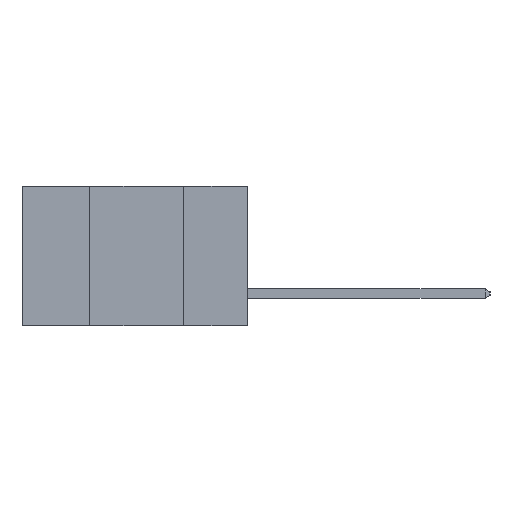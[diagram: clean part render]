
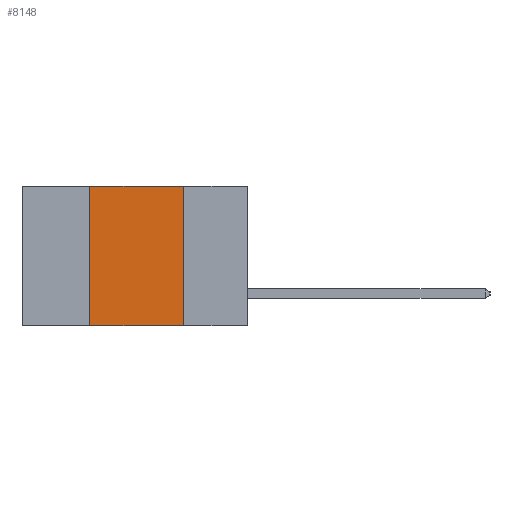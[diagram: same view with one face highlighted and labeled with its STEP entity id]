
A CAD part, left-side view. The second image highlights one B-rep face of the part: STEP entity #8148.
In plain terms, the highlighted planar face has unit normal (-1, 0, 0).
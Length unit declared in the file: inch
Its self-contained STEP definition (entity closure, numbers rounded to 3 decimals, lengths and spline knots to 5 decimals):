
#10 = EDGE_CURVE ( 'NONE', #8439, #10023, #8112, .T. ) ;
#141 = DIRECTION ( 'NONE',  ( 0., -1., 0. ) ) ;
#203 = CARTESIAN_POINT ( 'NONE',  ( 0., 0.17, -0.37 ) ) ;
#583 = CARTESIAN_POINT ( 'NONE',  ( 0., 0.6, -0.37 ) ) ;
#824 = AXIS2_PLACEMENT_3D ( 'NONE', #5664, #5415, #5399 ) ;
#1127 = ORIENTED_EDGE ( 'NONE', *, *, #3109, .F. ) ;
#1215 = ORIENTED_EDGE ( 'NONE', *, *, #1877, .F. ) ;
#1225 = ORIENTED_EDGE ( 'NONE', *, *, #10, .F. ) ;
#1273 = ORIENTED_EDGE ( 'NONE', *, *, #10413, .T. ) ;
#1379 = VERTEX_POINT ( 'NONE', #2957 ) ;
#1500 = LINE ( 'NONE', #583, #8401 ) ;
#1877 = EDGE_CURVE ( 'NONE', #10023, #7795, #3005, .T. ) ;
#2957 = CARTESIAN_POINT ( 'NONE',  ( 0., 0.17, -0.37 ) ) ;
#3005 = LINE ( 'NONE', #9600, #9531 ) ;
#3042 = CARTESIAN_POINT ( 'NONE',  ( 0., 0.17, 0. ) ) ;
#3109 = EDGE_CURVE ( 'NONE', #7795, #1379, #11236, .T. ) ;
#3281 = FACE_OUTER_BOUND ( 'NONE', #5167, .T. ) ;
#4810 = CARTESIAN_POINT ( 'NONE',  ( 0., 0.42, -0.37 ) ) ;
#5040 = DIRECTION ( 'NONE',  ( 0., 0., -1. ) ) ;
#5167 = EDGE_LOOP ( 'NONE', ( #1127, #1215, #1225, #1273 ) ) ;
#5399 = DIRECTION ( 'NONE',  ( 0., 0., -1. ) ) ;
#5415 = DIRECTION ( 'NONE',  ( 1., 0., 0. ) ) ;
#5664 = CARTESIAN_POINT ( 'NONE',  ( 0., 0.6, 0. ) ) ;
#5735 = PLANE ( 'NONE',  #824 ) ;
#5798 = VECTOR ( 'NONE', #6087, 39.37008 ) ;
#6087 = DIRECTION ( 'NONE',  ( 0., 0., 1. ) ) ;
#6803 = VECTOR ( 'NONE', #5040, 39.37008 ) ;
#7006 = CARTESIAN_POINT ( 'NONE',  ( 0., 0.42, 0. ) ) ;
#7795 = VERTEX_POINT ( 'NONE', #3042 ) ;
#8112 = LINE ( 'NONE', #4810, #5798 ) ;
#8148 = ADVANCED_FACE ( 'NONE', ( #3281 ), #5735, .F. ) ;
#8401 = VECTOR ( 'NONE', #141, 39.37008 ) ;
#8439 = VERTEX_POINT ( 'NONE', #10572 ) ;
#8731 = DIRECTION ( 'NONE',  ( 0., -1., 0. ) ) ;
#9531 = VECTOR ( 'NONE', #8731, 39.37008 ) ;
#9600 = CARTESIAN_POINT ( 'NONE',  ( 0., 0.6, 0. ) ) ;
#10023 = VERTEX_POINT ( 'NONE', #7006 ) ;
#10413 = EDGE_CURVE ( 'NONE', #8439, #1379, #1500, .T. ) ;
#10572 = CARTESIAN_POINT ( 'NONE',  ( 0., 0.42, -0.37 ) ) ;
#11236 = LINE ( 'NONE', #203, #6803 ) ;
